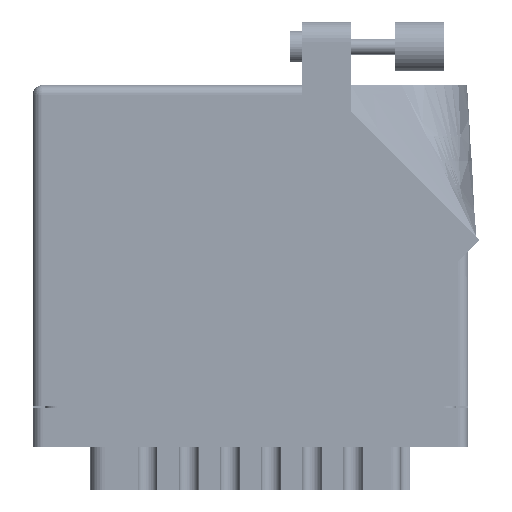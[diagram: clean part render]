
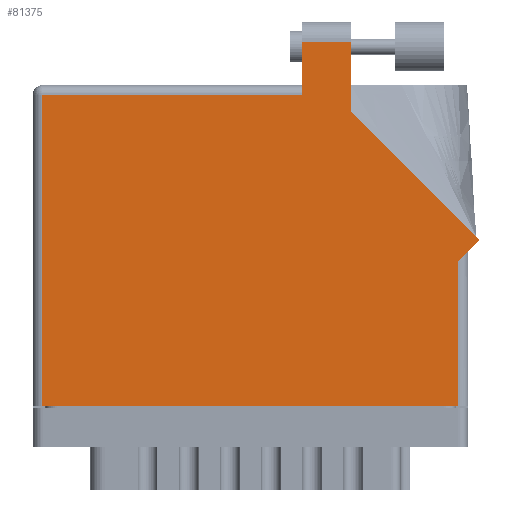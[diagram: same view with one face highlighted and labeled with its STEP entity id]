
A CAD part, front view. The second image highlights one B-rep face of the part: STEP entity #81375.
In plain terms, the highlighted face is planar.
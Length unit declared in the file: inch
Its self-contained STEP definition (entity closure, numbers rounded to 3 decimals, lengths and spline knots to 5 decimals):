
#184 = EDGE_CURVE ( 'NONE', #91704, #71206, #21469, .T. ) ;
#4199 = LINE ( 'NONE', #10097, #25652 ) ;
#5926 = EDGE_CURVE ( 'NONE', #30066, #91704, #67019, .T. ) ;
#7439 = DIRECTION ( 'NONE',  ( -1., 0., 0. ) ) ;
#8168 = EDGE_CURVE ( 'NONE', #55719, #66447, #37906, .T. ) ;
#8379 = DIRECTION ( 'NONE',  ( 0., 0., -1. ) ) ;
#10097 = CARTESIAN_POINT ( 'NONE',  ( 2.012, 1.86442, 0. ) ) ;
#10945 = CARTESIAN_POINT ( 'NONE',  ( 2.693, 0., 0. ) ) ;
#11408 = EDGE_CURVE ( 'NONE', #31332, #33083, #46718, .T. ) ;
#11581 = ORIENTED_EDGE ( 'NONE', *, *, #184, .T. ) ;
#14487 = VERTEX_POINT ( 'NONE', #68000 ) ;
#16316 = ORIENTED_EDGE ( 'NONE', *, *, #11408, .T. ) ;
#20533 = VECTOR ( 'NONE', #66964, 39.37008 ) ;
#21469 = LINE ( 'NONE', #64996, #46861 ) ;
#21539 = CARTESIAN_POINT ( 'NONE',  ( 1.705, 2.305, 0. ) ) ;
#23483 = VECTOR ( 'NONE', #72626, 39.37008 ) ;
#23694 = EDGE_CURVE ( 'NONE', #33083, #25760, #31646, .T. ) ;
#24246 = DIRECTION ( 'NONE',  ( -1., 0., 0. ) ) ;
#24789 = LINE ( 'NONE', #68798, #30450 ) ;
#25652 = VECTOR ( 'NONE', #69757, 39.37008 ) ;
#25760 = VERTEX_POINT ( 'NONE', #67337 ) ;
#27768 = CARTESIAN_POINT ( 'NONE',  ( 2.012, 1.86442, 0. ) ) ;
#28401 = CARTESIAN_POINT ( 'NONE',  ( 2.755, 0.98, 0. ) ) ;
#30066 = VERTEX_POINT ( 'NONE', #59728 ) ;
#30450 = VECTOR ( 'NONE', #62915, 39.37008 ) ;
#31049 = DIRECTION ( 'NONE',  ( 1., 0., 0. ) ) ;
#31332 = VERTEX_POINT ( 'NONE', #68038 ) ;
#31428 = ORIENTED_EDGE ( 'NONE', *, *, #91254, .T. ) ;
#31646 = LINE ( 'NONE', #61507, #89782 ) ;
#33083 = VERTEX_POINT ( 'NONE', #21539 ) ;
#33205 = ORIENTED_EDGE ( 'NONE', *, *, #83917, .T. ) ;
#34905 = EDGE_CURVE ( 'NONE', #25760, #14487, #24789, .T. ) ;
#35711 = DIRECTION ( 'NONE',  ( 0.707, 0.707, 0. ) ) ;
#37906 = LINE ( 'NONE', #67758, #76667 ) ;
#38061 = ORIENTED_EDGE ( 'NONE', *, *, #71417, .T. ) ;
#38280 = VECTOR ( 'NONE', #24246, 39.37008 ) ;
#38890 = CARTESIAN_POINT ( 'NONE',  ( 1.705, 2.305, 0. ) ) ;
#45383 = CARTESIAN_POINT ( 'NONE',  ( 0.062, 0., 0. ) ) ;
#45539 = FACE_OUTER_BOUND ( 'NONE', #91564, .T. ) ;
#46477 = ORIENTED_EDGE ( 'NONE', *, *, #23694, .T. ) ;
#46718 = LINE ( 'NONE', #38890, #38280 ) ;
#46861 = VECTOR ( 'NONE', #88399, 39.37008 ) ;
#48866 = ORIENTED_EDGE ( 'NONE', *, *, #34905, .T. ) ;
#55719 = VERTEX_POINT ( 'NONE', #45383 ) ;
#58933 = CARTESIAN_POINT ( 'NONE',  ( 2.693, 0.98, 0. ) ) ;
#59728 = CARTESIAN_POINT ( 'NONE',  ( 2.693, 0.918, 0. ) ) ;
#61507 = CARTESIAN_POINT ( 'NONE',  ( 1.705, 2.03, 0. ) ) ;
#62915 = DIRECTION ( 'NONE',  ( -1., 0., 0. ) ) ;
#63388 = ORIENTED_EDGE ( 'NONE', *, *, #8168, .T. ) ;
#64996 = CARTESIAN_POINT ( 'NONE',  ( 2.82571, 1.05071, 0. ) ) ;
#65034 = LINE ( 'NONE', #94811, #20533 ) ;
#66447 = VERTEX_POINT ( 'NONE', #10945 ) ;
#66964 = DIRECTION ( 'NONE',  ( 0., -1., 0. ) ) ;
#67019 = LINE ( 'NONE', #28401, #76599 ) ;
#67337 = CARTESIAN_POINT ( 'NONE',  ( 1.705, 1.968, 0. ) ) ;
#67758 = CARTESIAN_POINT ( 'NONE',  ( 0., 0., 0. ) ) ;
#68000 = CARTESIAN_POINT ( 'NONE',  ( 0.062, 1.968, 0. ) ) ;
#68038 = CARTESIAN_POINT ( 'NONE',  ( 2.012, 2.305, 0. ) ) ;
#68798 = CARTESIAN_POINT ( 'NONE',  ( 0., 1.968, 0. ) ) ;
#69757 = DIRECTION ( 'NONE',  ( 0., 1., 0. ) ) ;
#71206 = VERTEX_POINT ( 'NONE', #27768 ) ;
#71417 = EDGE_CURVE ( 'NONE', #71206, #31332, #4199, .T. ) ;
#72626 = DIRECTION ( 'NONE',  ( 0., 1., 0. ) ) ;
#72632 = ORIENTED_EDGE ( 'NONE', *, *, #5926, .T. ) ;
#75352 = CARTESIAN_POINT ( 'NONE',  ( 0., 2.03, 0. ) ) ;
#76599 = VECTOR ( 'NONE', #35711, 39.37008 ) ;
#76667 = VECTOR ( 'NONE', #31049, 39.37008 ) ;
#80840 = AXIS2_PLACEMENT_3D ( 'NONE', #75352, #8379, #7439 ) ;
#81375 = ADVANCED_FACE ( 'NONE', ( #45539 ), #89044, .F. ) ;
#83917 = EDGE_CURVE ( 'NONE', #66447, #30066, #95539, .T. ) ;
#83965 = DIRECTION ( 'NONE',  ( 0., -1., 0. ) ) ;
#88399 = DIRECTION ( 'NONE',  ( -0.707, 0.707, 0. ) ) ;
#89044 = PLANE ( 'NONE',  #80840 ) ;
#89782 = VECTOR ( 'NONE', #83965, 39.37008 ) ;
#91254 = EDGE_CURVE ( 'NONE', #14487, #55719, #65034, .T. ) ;
#91564 = EDGE_LOOP ( 'NONE', ( #38061, #16316, #46477, #48866, #31428, #63388, #33205, #72632, #11581 ) ) ;
#91704 = VERTEX_POINT ( 'NONE', #94215 ) ;
#94215 = CARTESIAN_POINT ( 'NONE',  ( 2.82571, 1.05071, 0. ) ) ;
#94811 = CARTESIAN_POINT ( 'NONE',  ( 0.062, 0., 0. ) ) ;
#95539 = LINE ( 'NONE', #58933, #23483 ) ;
